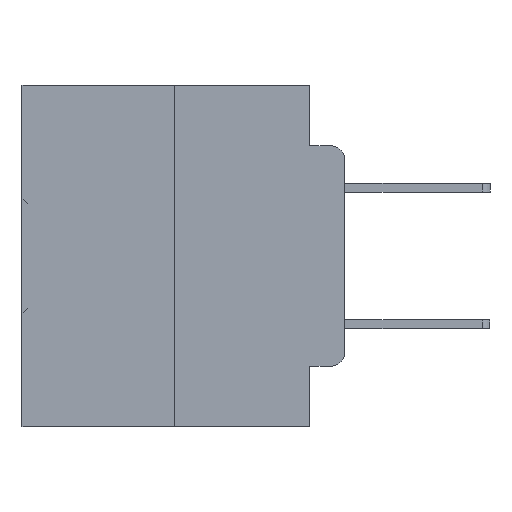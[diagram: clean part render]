
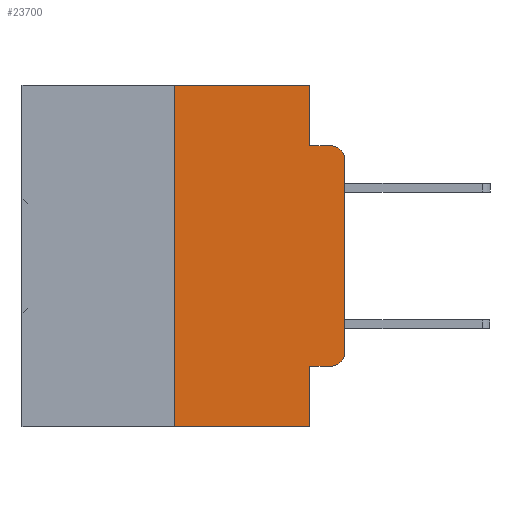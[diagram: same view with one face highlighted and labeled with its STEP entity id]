
A CAD part, left-side view. The second image highlights one B-rep face of the part: STEP entity #23700.
In plain terms, the highlighted planar face has unit normal (-1, 0, 0).
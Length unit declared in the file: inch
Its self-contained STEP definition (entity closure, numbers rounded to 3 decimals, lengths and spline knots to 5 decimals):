
#34 = VECTOR ( 'NONE', #10182, 39.37008 ) ;
#385 = CARTESIAN_POINT ( 'NONE',  ( 0., 0., 0. ) ) ;
#702 = CARTESIAN_POINT ( 'NONE',  ( 0., 0.02, -0.3915 ) ) ;
#833 = CARTESIAN_POINT ( 'NONE',  ( 0., 0.473, 0. ) ) ;
#1650 = EDGE_CURVE ( 'NONE', #13827, #20137, #26605, .T. ) ;
#1674 = DIRECTION ( 'NONE',  ( 0., 0., -1. ) ) ;
#2045 = CARTESIAN_POINT ( 'NONE',  ( 0., 0.051, 0. ) ) ;
#2050 = CARTESIAN_POINT ( 'NONE',  ( 0., 0.051, -0.5 ) ) ;
#3321 = EDGE_LOOP ( 'NONE', ( #22728, #10722, #22219, #25415, #22361, #23185, #15384, #14539, #15324, #14699 ) ) ;
#3583 = DIRECTION ( 'NONE',  ( 0., 0., -1. ) ) ;
#5675 = CARTESIAN_POINT ( 'NONE',  ( 0., 0.051, 0. ) ) ;
#7077 = CARTESIAN_POINT ( 'NONE',  ( 0., 0.051, 0. ) ) ;
#7093 = LINE ( 'NONE', #5675, #35813 ) ;
#7273 = VECTOR ( 'NONE', #29028, 39.37008 ) ;
#7404 = FACE_OUTER_BOUND ( 'NONE', #3321, .T. ) ;
#9175 = DIRECTION ( 'NONE',  ( 0., 0., -1. ) ) ;
#9362 = VERTEX_POINT ( 'NONE', #25543 ) ;
#9434 = CIRCLE ( 'NONE', #17470, 0.02 ) ;
#9585 = VECTOR ( 'NONE', #20172, 39.37008 ) ;
#9928 = DIRECTION ( 'NONE',  ( 0., 0., -1. ) ) ;
#10182 = DIRECTION ( 'NONE',  ( 0., -1., 0. ) ) ;
#10722 = ORIENTED_EDGE ( 'NONE', *, *, #16832, .T. ) ;
#11203 = EDGE_CURVE ( 'NONE', #31509, #19976, #7093, .T. ) ;
#11316 = LINE ( 'NONE', #26318, #26171 ) ;
#11919 = VERTEX_POINT ( 'NONE', #2050 ) ;
#12102 = LINE ( 'NONE', #7077, #31725 ) ;
#13827 = VERTEX_POINT ( 'NONE', #21538 ) ;
#14539 = ORIENTED_EDGE ( 'NONE', *, *, #36035, .F. ) ;
#14699 = ORIENTED_EDGE ( 'NONE', *, *, #28767, .T. ) ;
#14721 = CARTESIAN_POINT ( 'NONE',  ( 0., 0.473, 0. ) ) ;
#14735 = CARTESIAN_POINT ( 'NONE',  ( 0., 0.02, -0.0885 ) ) ;
#14750 = VERTEX_POINT ( 'NONE', #22573 ) ;
#14799 = LINE ( 'NONE', #833, #7273 ) ;
#14971 = EDGE_CURVE ( 'NONE', #19976, #26988, #11316, .T. ) ;
#15142 = LINE ( 'NONE', #16065, #34 ) ;
#15166 = VERTEX_POINT ( 'NONE', #16038 ) ;
#15324 = ORIENTED_EDGE ( 'NONE', *, *, #34260, .T. ) ;
#15384 = ORIENTED_EDGE ( 'NONE', *, *, #26658, .T. ) ;
#16025 = DIRECTION ( 'NONE',  ( 0., 0., 1. ) ) ;
#16038 = CARTESIAN_POINT ( 'NONE',  ( 0., 0.051, -0.4115 ) ) ;
#16065 = CARTESIAN_POINT ( 'NONE',  ( 0., 0.473, -0.5 ) ) ;
#16832 = EDGE_CURVE ( 'NONE', #29518, #26988, #9434, .T. ) ;
#17470 = AXIS2_PLACEMENT_3D ( 'NONE', #35153, #18626, #1674 ) ;
#17730 = CARTESIAN_POINT ( 'NONE',  ( 0., 0.051, -0.0885 ) ) ;
#17986 = CARTESIAN_POINT ( 'NONE',  ( 0., 0., -0.1085 ) ) ;
#18626 = DIRECTION ( 'NONE',  ( -1., 0., 0. ) ) ;
#18723 = LINE ( 'NONE', #26922, #25277 ) ;
#18940 = AXIS2_PLACEMENT_3D ( 'NONE', #702, #20491, #3583 ) ;
#19209 = VECTOR ( 'NONE', #16025, 39.37008 ) ;
#19976 = VERTEX_POINT ( 'NONE', #17730 ) ;
#20137 = VERTEX_POINT ( 'NONE', #21160 ) ;
#20172 = DIRECTION ( 'NONE',  ( 0., 0., 1. ) ) ;
#20491 = DIRECTION ( 'NONE',  ( -1., 0., 0. ) ) ;
#20746 = DIRECTION ( 'NONE',  ( 0., -1., 0. ) ) ;
#21160 = CARTESIAN_POINT ( 'NONE',  ( 0., 0.25, 0. ) ) ;
#21538 = CARTESIAN_POINT ( 'NONE',  ( 0., 0.25, -0.5 ) ) ;
#22219 = ORIENTED_EDGE ( 'NONE', *, *, #14971, .F. ) ;
#22361 = ORIENTED_EDGE ( 'NONE', *, *, #34114, .F. ) ;
#22573 = CARTESIAN_POINT ( 'NONE',  ( 0., 0.02, -0.4115 ) ) ;
#22728 = ORIENTED_EDGE ( 'NONE', *, *, #24317, .T. ) ;
#23185 = ORIENTED_EDGE ( 'NONE', *, *, #1650, .F. ) ;
#23700 = ADVANCED_FACE ( 'NONE', ( #7404 ), #34125, .F. ) ;
#24317 = EDGE_CURVE ( 'NONE', #9362, #29518, #31016, .T. ) ;
#24432 = AXIS2_PLACEMENT_3D ( 'NONE', #14721, #25934, #9175 ) ;
#25277 = VECTOR ( 'NONE', #29741, 39.37008 ) ;
#25415 = ORIENTED_EDGE ( 'NONE', *, *, #11203, .F. ) ;
#25543 = CARTESIAN_POINT ( 'NONE',  ( 0., 0., -0.3915 ) ) ;
#25934 = DIRECTION ( 'NONE',  ( 1., 0., 0. ) ) ;
#26171 = VECTOR ( 'NONE', #20746, 39.37008 ) ;
#26318 = CARTESIAN_POINT ( 'NONE',  ( 0., 0.051, -0.0885 ) ) ;
#26605 = LINE ( 'NONE', #28528, #19209 ) ;
#26658 = EDGE_CURVE ( 'NONE', #13827, #11919, #15142, .T. ) ;
#26922 = CARTESIAN_POINT ( 'NONE',  ( 0., 0.051, -0.4115 ) ) ;
#26988 = VERTEX_POINT ( 'NONE', #14735 ) ;
#28528 = CARTESIAN_POINT ( 'NONE',  ( 0., 0.25, 0. ) ) ;
#28767 = EDGE_CURVE ( 'NONE', #14750, #9362, #30430, .T. ) ;
#29028 = DIRECTION ( 'NONE',  ( 0., -1., 0. ) ) ;
#29518 = VERTEX_POINT ( 'NONE', #17986 ) ;
#29741 = DIRECTION ( 'NONE',  ( 0., -1., 0. ) ) ;
#30430 = CIRCLE ( 'NONE', #18940, 0.02 ) ;
#31016 = LINE ( 'NONE', #385, #9585 ) ;
#31509 = VERTEX_POINT ( 'NONE', #2045 ) ;
#31725 = VECTOR ( 'NONE', #9928, 39.37008 ) ;
#33660 = DIRECTION ( 'NONE',  ( 0., 0., -1. ) ) ;
#34114 = EDGE_CURVE ( 'NONE', #20137, #31509, #14799, .T. ) ;
#34125 = PLANE ( 'NONE',  #24432 ) ;
#34260 = EDGE_CURVE ( 'NONE', #15166, #14750, #18723, .T. ) ;
#35153 = CARTESIAN_POINT ( 'NONE',  ( 0., 0.02, -0.1085 ) ) ;
#35813 = VECTOR ( 'NONE', #33660, 39.37008 ) ;
#36035 = EDGE_CURVE ( 'NONE', #15166, #11919, #12102, .T. ) ;
